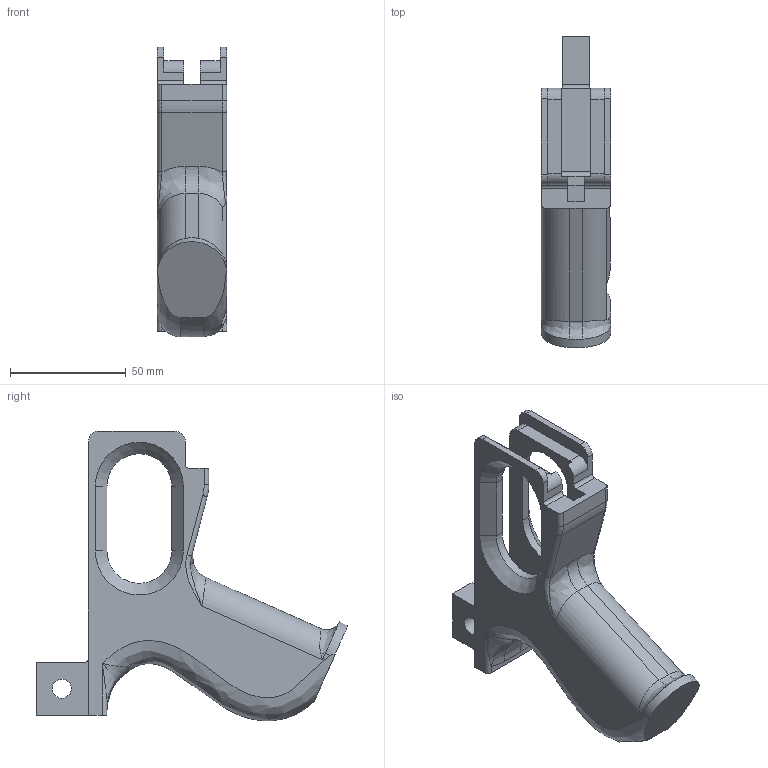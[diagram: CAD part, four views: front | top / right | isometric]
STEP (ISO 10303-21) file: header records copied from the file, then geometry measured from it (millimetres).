
FILE_DESCRIPTION((''),'2;1');
FILE_NAME('PM522Grip2.stp','2015-10-01T18:16:05',('JamesRPatrick'),(''),'Autodesk Inventor 2012','Autodesk Inventor 2012','');
FILE_SCHEMA(('AUTOMOTIVE_DESIGN { 1 0 10303 214 1 1 1 1 }'));
Length unit declared in the file: millimetre
Products named in the file (1): PM522Grip2
Bounding box: 30 x 134.71 x 125.22 mm (x, y, z)
Volume: 107012.9 mm3; surface area: 37171 mm2
Topology: 1 solids, 1 shells, 110 faces, 305 edges, 192 vertices
Faces by surface type: plane 59, cylinder 28, bspline 17, cone 4, torus 2
Full cylindrical faces by diameter (mm): 8.2 x1
Entity records: 4816 total; most frequent: CARTESIAN_POINT 2051, ORIENTED_EDGE 598, DIRECTION 522, EDGE_CURVE 299, VERTEX_POINT 192, VECTOR 188, LINE 188, AXIS2_PLACEMENT_3D 167
